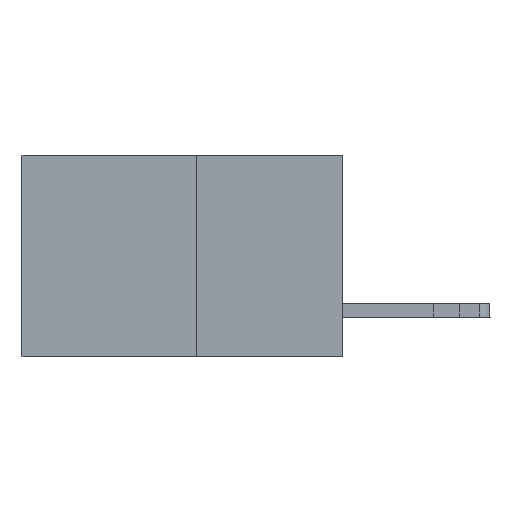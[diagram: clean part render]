
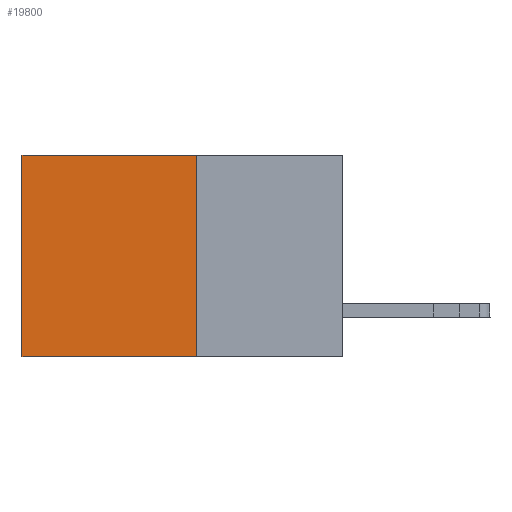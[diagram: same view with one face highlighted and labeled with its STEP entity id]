
A CAD part, left-side view. The second image highlights one B-rep face of the part: STEP entity #19800.
In plain terms, the highlighted planar face has unit normal (-1, 0, 0).
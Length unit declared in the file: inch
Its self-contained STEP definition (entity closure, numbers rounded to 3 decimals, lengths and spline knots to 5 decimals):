
#24 = EDGE_CURVE ( 'NONE', #17234, #26121, #17995, .T. ) ;
#215 = DIRECTION ( 'NONE',  ( 0., 1., 0. ) ) ;
#3126 = DIRECTION ( 'NONE',  ( 0., 0., -1. ) ) ;
#6013 = EDGE_CURVE ( 'NONE', #17234, #25221, #22841, .T. ) ;
#6216 = PLANE ( 'NONE',  #26268 ) ;
#6507 = CARTESIAN_POINT ( 'NONE',  ( 0.277, 0.59, -0.37 ) ) ;
#6524 = CARTESIAN_POINT ( 'NONE',  ( 0.277, 0.27, 0. ) ) ;
#7006 = EDGE_CURVE ( 'NONE', #26121, #20064, #7644, .T. ) ;
#7335 = EDGE_CURVE ( 'NONE', #25221, #20064, #13798, .T. ) ;
#7644 = LINE ( 'NONE', #16855, #20157 ) ;
#8313 = VECTOR ( 'NONE', #27539, 39.37008 ) ;
#8816 = ORIENTED_EDGE ( 'NONE', *, *, #7335, .F. ) ;
#10590 = DIRECTION ( 'NONE',  ( 1., 0., 0. ) ) ;
#12379 = CARTESIAN_POINT ( 'NONE',  ( 0.277, 0.59, 0. ) ) ;
#12603 = CARTESIAN_POINT ( 'NONE',  ( 0.277, 0.27, -0.37 ) ) ;
#13798 = LINE ( 'NONE', #22992, #20237 ) ;
#14820 = ORIENTED_EDGE ( 'NONE', *, *, #24, .T. ) ;
#15704 = ORIENTED_EDGE ( 'NONE', *, *, #7006, .T. ) ;
#16855 = CARTESIAN_POINT ( 'NONE',  ( 0.277, 0.59, -0.37 ) ) ;
#16950 = FACE_OUTER_BOUND ( 'NONE', #27647, .T. ) ;
#17234 = VERTEX_POINT ( 'NONE', #24159 ) ;
#17995 = LINE ( 'NONE', #6524, #18102 ) ;
#18102 = VECTOR ( 'NONE', #24774, 39.37008 ) ;
#19800 = ADVANCED_FACE ( 'NONE', ( #16950 ), #6216, .F. ) ;
#20064 = VERTEX_POINT ( 'NONE', #6507 ) ;
#20157 = VECTOR ( 'NONE', #3126, 39.37008 ) ;
#20237 = VECTOR ( 'NONE', #215, 39.37008 ) ;
#20584 = CARTESIAN_POINT ( 'NONE',  ( 0.277, 0.27, -0.37 ) ) ;
#22841 = LINE ( 'NONE', #20584, #8313 ) ;
#22885 = ORIENTED_EDGE ( 'NONE', *, *, #6013, .F. ) ;
#22992 = CARTESIAN_POINT ( 'NONE',  ( 0.277, 0.27, -0.37 ) ) ;
#24159 = CARTESIAN_POINT ( 'NONE',  ( 0.277, 0.27, 0. ) ) ;
#24774 = DIRECTION ( 'NONE',  ( 0., 1., 0. ) ) ;
#25221 = VERTEX_POINT ( 'NONE', #12603 ) ;
#26121 = VERTEX_POINT ( 'NONE', #12379 ) ;
#26268 = AXIS2_PLACEMENT_3D ( 'NONE', #26601, #10590, #29013 ) ;
#26601 = CARTESIAN_POINT ( 'NONE',  ( 0.277, 0.27, -0.37 ) ) ;
#27539 = DIRECTION ( 'NONE',  ( 0., 0., -1. ) ) ;
#27647 = EDGE_LOOP ( 'NONE', ( #15704, #8816, #22885, #14820 ) ) ;
#29013 = DIRECTION ( 'NONE',  ( 0., 0., -1. ) ) ;
